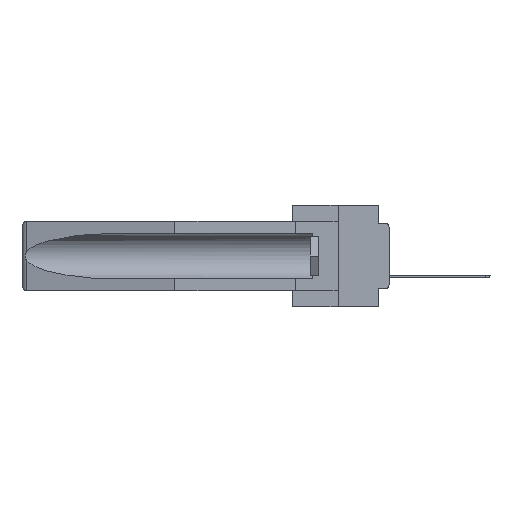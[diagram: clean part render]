
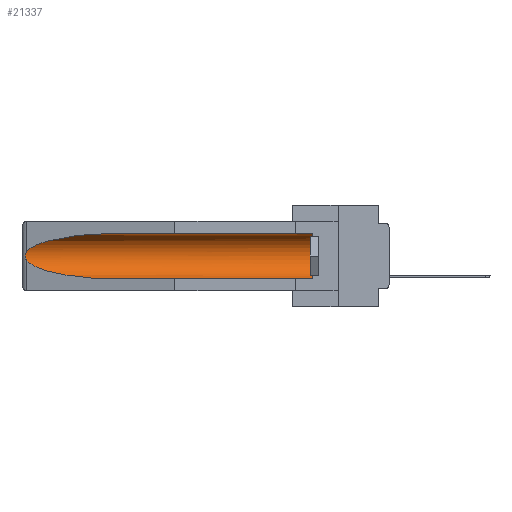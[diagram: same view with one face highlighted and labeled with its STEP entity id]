
A CAD part, left-side view. The second image highlights one B-rep face of the part: STEP entity #21337.
In plain terms, the highlighted cylindrical face has radius 2.857 mm (diameter 5.715 mm), a partial arc.
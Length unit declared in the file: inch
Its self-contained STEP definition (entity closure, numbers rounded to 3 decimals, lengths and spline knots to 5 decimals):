
#213 = ORIENTED_EDGE ( 'NONE', *, *, #11909, .F. ) ;
#1675 = CARTESIAN_POINT ( 'NONE',  ( 0.155, 1.07973, -0.059 ) ) ;
#1909 = CARTESIAN_POINT ( 'NONE',  ( 0.155, -0.30754, -0.059 ) ) ;
#2283 = FACE_OUTER_BOUND ( 'NONE', #13076, .T. ) ;
#2366 = AXIS2_PLACEMENT_3D ( 'NONE', #9553, #5096, #17622 ) ;
#3213 = AXIS2_PLACEMENT_3D ( 'NONE', #25182, #12680, #30449 ) ;
#3854 = VERTEX_POINT ( 'NONE', #26258 ) ;
#3923 = CARTESIAN_POINT ( 'NONE',  ( 0.21114, 1.30732, -0.284 ) ) ;
#5096 = DIRECTION ( 'NONE',  ( 0., -1., 0. ) ) ;
#5249 = CYLINDRICAL_SURFACE ( 'NONE', #3213, 0.1125 ) ;
#5927 = CARTESIAN_POINT ( 'NONE',  ( 0.2675, 1.53308, -0.16763 ) ) ;
#6422 = ORIENTED_EDGE ( 'NONE', *, *, #24499, .T. ) ;
#6526 = DIRECTION ( 'NONE',  ( 0., 1., 0. ) ) ;
#6547 = CARTESIAN_POINT ( 'NONE',  ( 0.26597, 1.5296, -0.19026 ) ) ;
#6898 = VECTOR ( 'NONE', #6526, 39.37008 ) ;
#8495 = EDGE_CURVE ( 'NONE', #3854, #29105, #9659, .T. ) ;
#8649 = VERTEX_POINT ( 'NONE', #29912 ) ;
#8735 =( BOUNDED_CURVE ( )  B_SPLINE_CURVE ( 3, ( #26495, #18603, #3923, #28635 ),
 .UNSPECIFIED., .F., .T. ) 
 B_SPLINE_CURVE_WITH_KNOTS ( ( 4, 4 ),
 ( 0.1948, 1.5708 ),
 .UNSPECIFIED. ) 
 CURVE ( )  GEOMETRIC_REPRESENTATION_ITEM ( )  RATIONAL_B_SPLINE_CURVE ( ( 1., 0.848, 0.848, 1. ) ) 
 REPRESENTATION_ITEM ( '' )  );
#9366 = ORIENTED_EDGE ( 'NONE', *, *, #18252, .T. ) ;
#9553 = CARTESIAN_POINT ( 'NONE',  ( 0.155, 0.126, -0.1715 ) ) ;
#9659 = LINE ( 'NONE', #1909, #6898 ) ;
#9692 = VECTOR ( 'NONE', #14409, 39.37008 ) ;
#9787 = VERTEX_POINT ( 'NONE', #26999 ) ;
#10783 = CIRCLE ( 'NONE', #2366, 0.1125 ) ;
#11177 = CARTESIAN_POINT ( 'NONE',  ( 0.26654, 1.53092, -0.15636 ) ) ;
#11396 = CARTESIAN_POINT ( 'NONE',  ( 0.21114, 1.30732, -0.059 ) ) ;
#11909 = EDGE_CURVE ( 'NONE', #8649, #23497, #29231, .T. ) ;
#12680 = DIRECTION ( 'NONE',  ( 0., 1., 0. ) ) ;
#13076 = EDGE_LOOP ( 'NONE', ( #9366, #24580, #19380, #213, #6422, #28819 ) ) ;
#13649 = CARTESIAN_POINT ( 'NONE',  ( 0.26537, 1.52718, -0.19328 ) ) ;
#14409 = DIRECTION ( 'NONE',  ( 0., 1., 0. ) ) ;
#15640 = EDGE_CURVE ( 'NONE', #26001, #9787, #23427, .T. ) ;
#15725 = EDGE_CURVE ( 'NONE', #9787, #23497, #8735, .T. ) ;
#16550 = CARTESIAN_POINT ( 'NONE',  ( 0.155, 1.07973, -0.284 ) ) ;
#17622 = DIRECTION ( 'NONE',  ( 0., 0., 1. ) ) ;
#18252 = EDGE_CURVE ( 'NONE', #29105, #26001, #28939, .T. ) ;
#18603 = CARTESIAN_POINT ( 'NONE',  ( 0.25451, 1.48313, -0.24835 ) ) ;
#19087 = CARTESIAN_POINT ( 'NONE',  ( 0.26597, 1.52961, -0.15275 ) ) ;
#19380 = ORIENTED_EDGE ( 'NONE', *, *, #15725, .T. ) ;
#21337 = ADVANCED_FACE ( 'NONE', ( #2283 ), #5249, .F. ) ;
#23427 = B_SPLINE_CURVE_WITH_KNOTS ( 'NONE', 3,
 ( #28792, #19087, #11177, #29125, #5927, #31271, #24200, #24031, #6547, #13649 ),
 .UNSPECIFIED., .F., .F.,
 ( 4, 2, 2, 2, 4 ),
 ( 0., 0.00029, 0.00058, 0.00087, 0.00117 ),
 .UNSPECIFIED. ) ;
#23497 = VERTEX_POINT ( 'NONE', #16550 ) ;
#24031 = CARTESIAN_POINT ( 'NONE',  ( 0.26655, 1.53094, -0.18657 ) ) ;
#24200 = CARTESIAN_POINT ( 'NONE',  ( 0.2673, 1.53269, -0.17917 ) ) ;
#24499 = EDGE_CURVE ( 'NONE', #8649, #3854, #10783, .T. ) ;
#24580 = ORIENTED_EDGE ( 'NONE', *, *, #15640, .T. ) ;
#25182 = CARTESIAN_POINT ( 'NONE',  ( 0.155, -0.30754, -0.1715 ) ) ;
#26001 = VERTEX_POINT ( 'NONE', #27349 ) ;
#26258 = CARTESIAN_POINT ( 'NONE',  ( 0.155, 0.126, -0.059 ) ) ;
#26495 = CARTESIAN_POINT ( 'NONE',  ( 0.26537, 1.52718, -0.19328 ) ) ;
#26999 = CARTESIAN_POINT ( 'NONE',  ( 0.26537, 1.52718, -0.19328 ) ) ;
#27349 = CARTESIAN_POINT ( 'NONE',  ( 0.26537, 1.52718, -0.14972 ) ) ;
#28635 = CARTESIAN_POINT ( 'NONE',  ( 0.155, 1.07973, -0.284 ) ) ;
#28792 = CARTESIAN_POINT ( 'NONE',  ( 0.26537, 1.52718, -0.14972 ) ) ;
#28819 = ORIENTED_EDGE ( 'NONE', *, *, #8495, .T. ) ;
#28939 =( BOUNDED_CURVE ( )  B_SPLINE_CURVE ( 3, ( #1675, #11396, #31673, #29184 ),
 .UNSPECIFIED., .F., .T. ) 
 B_SPLINE_CURVE_WITH_KNOTS ( ( 4, 4 ),
 ( 4.71239, 6.08839 ),
 .UNSPECIFIED. ) 
 CURVE ( )  GEOMETRIC_REPRESENTATION_ITEM ( )  RATIONAL_B_SPLINE_CURVE ( ( 1., 0.848, 0.848, 1. ) ) 
 REPRESENTATION_ITEM ( '' )  );
#29074 = CARTESIAN_POINT ( 'NONE',  ( 0.155, -0.30754, -0.284 ) ) ;
#29105 = VERTEX_POINT ( 'NONE', #30636 ) ;
#29125 = CARTESIAN_POINT ( 'NONE',  ( 0.2673, 1.5327, -0.16383 ) ) ;
#29184 = CARTESIAN_POINT ( 'NONE',  ( 0.26537, 1.52718, -0.14972 ) ) ;
#29231 = LINE ( 'NONE', #29074, #9692 ) ;
#29912 = CARTESIAN_POINT ( 'NONE',  ( 0.155, 0.126, -0.284 ) ) ;
#30449 = DIRECTION ( 'NONE',  ( 0., 0., 1. ) ) ;
#30636 = CARTESIAN_POINT ( 'NONE',  ( 0.155, 1.07973, -0.059 ) ) ;
#31271 = CARTESIAN_POINT ( 'NONE',  ( 0.2675, 1.53308, -0.17534 ) ) ;
#31673 = CARTESIAN_POINT ( 'NONE',  ( 0.25451, 1.48313, -0.09465 ) ) ;
